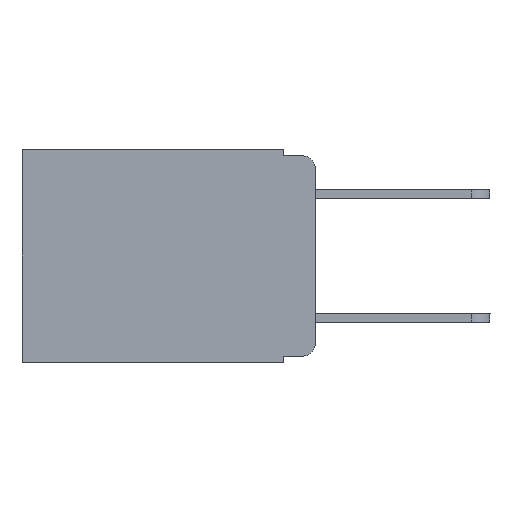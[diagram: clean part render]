
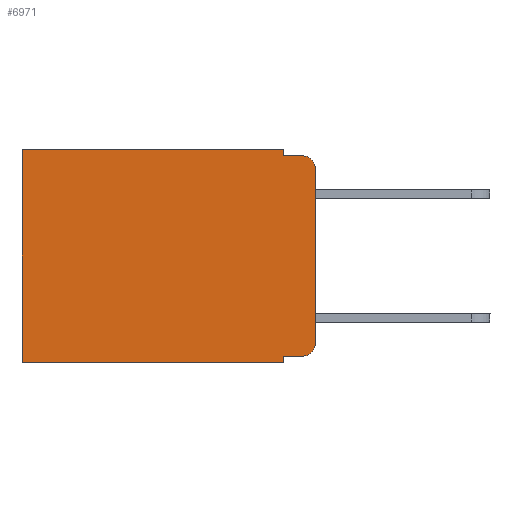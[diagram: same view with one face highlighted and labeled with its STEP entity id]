
A CAD part, left-side view. The second image highlights one B-rep face of the part: STEP entity #6971.
In plain terms, the highlighted planar face has unit normal (-1, 0, 0).
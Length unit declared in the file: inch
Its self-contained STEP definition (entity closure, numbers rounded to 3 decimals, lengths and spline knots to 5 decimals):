
#19 = EDGE_LOOP ( 'NONE', ( #11309, #1333, #9382, #1086, #11175, #11782, #8486, #11681, #6198, #8059 ) ) ;
#22 = CARTESIAN_POINT ( 'NONE',  ( 0.298, 0., -0.343 ) ) ;
#275 = CARTESIAN_POINT ( 'NONE',  ( 0.298, 0., -0.03 ) ) ;
#276 = CARTESIAN_POINT ( 'NONE',  ( 0.298, 0.051, -0.01 ) ) ;
#746 = VERTEX_POINT ( 'NONE', #3378 ) ;
#762 = VECTOR ( 'NONE', #1900, 39.37008 ) ;
#803 = DIRECTION ( 'NONE',  ( -1., 0., 0. ) ) ;
#831 = EDGE_CURVE ( 'NONE', #10962, #7118, #8297, .T. ) ;
#869 = CARTESIAN_POINT ( 'NONE',  ( 0.298, 0.02, -0.313 ) ) ;
#1002 = AXIS2_PLACEMENT_3D ( 'NONE', #869, #2581, #2656 ) ;
#1045 = CARTESIAN_POINT ( 'NONE',  ( 0.298, 0.02, -0.333 ) ) ;
#1086 = ORIENTED_EDGE ( 'NONE', *, *, #831, .F. ) ;
#1136 = PLANE ( 'NONE',  #4852 ) ;
#1247 = DIRECTION ( 'NONE',  ( 0., 0., -1. ) ) ;
#1286 = CARTESIAN_POINT ( 'NONE',  ( 0.298, 0.051, 0. ) ) ;
#1333 = ORIENTED_EDGE ( 'NONE', *, *, #5876, .T. ) ;
#1400 = VECTOR ( 'NONE', #3873, 39.37008 ) ;
#1679 = EDGE_CURVE ( 'NONE', #10876, #7322, #10410, .T. ) ;
#1855 = EDGE_CURVE ( 'NONE', #4520, #7322, #10554, .T. ) ;
#1900 = DIRECTION ( 'NONE',  ( 0., -1., 0. ) ) ;
#2052 = CARTESIAN_POINT ( 'NONE',  ( 0.298, 0.051, -0.343 ) ) ;
#2349 = VERTEX_POINT ( 'NONE', #4841 ) ;
#2581 = DIRECTION ( 'NONE',  ( -1., 0., 0. ) ) ;
#2656 = DIRECTION ( 'NONE',  ( 0., 0., -1. ) ) ;
#2741 = VERTEX_POINT ( 'NONE', #5350 ) ;
#2748 = DIRECTION ( 'NONE',  ( 0., 0., -1. ) ) ;
#2796 = EDGE_CURVE ( 'NONE', #2349, #10876, #5764, .T. ) ;
#2834 = EDGE_CURVE ( 'NONE', #6179, #2741, #4621, .T. ) ;
#2961 = FACE_OUTER_BOUND ( 'NONE', #19, .T. ) ;
#3032 = DIRECTION ( 'NONE',  ( 0., -1., 0. ) ) ;
#3051 = CARTESIAN_POINT ( 'NONE',  ( 0.298, 0., 0. ) ) ;
#3378 = CARTESIAN_POINT ( 'NONE',  ( 0.298, 0.02, -0.01 ) ) ;
#3443 = VECTOR ( 'NONE', #5632, 39.37008 ) ;
#3483 = VECTOR ( 'NONE', #1247, 39.37008 ) ;
#3873 = DIRECTION ( 'NONE',  ( 0., 1., 0. ) ) ;
#4289 = VERTEX_POINT ( 'NONE', #10028 ) ;
#4406 = EDGE_CURVE ( 'NONE', #4289, #2741, #6688, .T. ) ;
#4520 = VERTEX_POINT ( 'NONE', #275 ) ;
#4621 = LINE ( 'NONE', #22, #9868 ) ;
#4659 = CARTESIAN_POINT ( 'NONE',  ( 0.298, 0.051, 0. ) ) ;
#4678 = VECTOR ( 'NONE', #3032, 39.37008 ) ;
#4841 = CARTESIAN_POINT ( 'NONE',  ( 0.298, 0.051, -0.333 ) ) ;
#4852 = AXIS2_PLACEMENT_3D ( 'NONE', #8411, #9332, #10132 ) ;
#4982 = CIRCLE ( 'NONE', #6581, 0.02 ) ;
#5005 = VECTOR ( 'NONE', #9446, 39.37008 ) ;
#5350 = CARTESIAN_POINT ( 'NONE',  ( 0.298, 0.473, -0.343 ) ) ;
#5472 = CARTESIAN_POINT ( 'NONE',  ( 0.298, 0., -0.313 ) ) ;
#5632 = DIRECTION ( 'NONE',  ( 0., 0., -1. ) ) ;
#5764 = LINE ( 'NONE', #8216, #762 ) ;
#5790 = CARTESIAN_POINT ( 'NONE',  ( 0.298, 0.051, 0. ) ) ;
#5876 = EDGE_CURVE ( 'NONE', #4520, #746, #4982, .T. ) ;
#6179 = VERTEX_POINT ( 'NONE', #2052 ) ;
#6198 = ORIENTED_EDGE ( 'NONE', *, *, #2796, .T. ) ;
#6223 = CARTESIAN_POINT ( 'NONE',  ( 0.298, 0.02, -0.03 ) ) ;
#6354 = LINE ( 'NONE', #9318, #1400 ) ;
#6581 = AXIS2_PLACEMENT_3D ( 'NONE', #6223, #803, #9908 ) ;
#6688 = LINE ( 'NONE', #10902, #3443 ) ;
#6971 = ADVANCED_FACE ( 'NONE', ( #2961 ), #1136, .F. ) ;
#7118 = VERTEX_POINT ( 'NONE', #11278 ) ;
#7322 = VERTEX_POINT ( 'NONE', #5472 ) ;
#8059 = ORIENTED_EDGE ( 'NONE', *, *, #1679, .T. ) ;
#8216 = CARTESIAN_POINT ( 'NONE',  ( 0.298, 0.051, -0.333 ) ) ;
#8297 = LINE ( 'NONE', #5790, #3483 ) ;
#8411 = CARTESIAN_POINT ( 'NONE',  ( 0.298, 0., 0. ) ) ;
#8486 = ORIENTED_EDGE ( 'NONE', *, *, #2834, .F. ) ;
#8487 = EDGE_CURVE ( 'NONE', #2349, #6179, #8607, .T. ) ;
#8607 = LINE ( 'NONE', #4659, #9886 ) ;
#9088 = LINE ( 'NONE', #276, #4678 ) ;
#9133 = DIRECTION ( 'NONE',  ( 0., 1., 0. ) ) ;
#9318 = CARTESIAN_POINT ( 'NONE',  ( 0.298, 0., 0. ) ) ;
#9332 = DIRECTION ( 'NONE',  ( 1., 0., 0. ) ) ;
#9382 = ORIENTED_EDGE ( 'NONE', *, *, #10163, .F. ) ;
#9446 = DIRECTION ( 'NONE',  ( 0., 0., -1. ) ) ;
#9868 = VECTOR ( 'NONE', #9133, 39.37008 ) ;
#9886 = VECTOR ( 'NONE', #2748, 39.37008 ) ;
#9908 = DIRECTION ( 'NONE',  ( 0., 0., -1. ) ) ;
#10028 = CARTESIAN_POINT ( 'NONE',  ( 0.298, 0.473, 0. ) ) ;
#10132 = DIRECTION ( 'NONE',  ( 0., 0., -1. ) ) ;
#10163 = EDGE_CURVE ( 'NONE', #7118, #746, #9088, .T. ) ;
#10410 = CIRCLE ( 'NONE', #1002, 0.02 ) ;
#10554 = LINE ( 'NONE', #3051, #5005 ) ;
#10876 = VERTEX_POINT ( 'NONE', #1045 ) ;
#10881 = EDGE_CURVE ( 'NONE', #10962, #4289, #6354, .T. ) ;
#10902 = CARTESIAN_POINT ( 'NONE',  ( 0.298, 0.473, 0. ) ) ;
#10962 = VERTEX_POINT ( 'NONE', #1286 ) ;
#11175 = ORIENTED_EDGE ( 'NONE', *, *, #10881, .T. ) ;
#11278 = CARTESIAN_POINT ( 'NONE',  ( 0.298, 0.051, -0.01 ) ) ;
#11309 = ORIENTED_EDGE ( 'NONE', *, *, #1855, .F. ) ;
#11681 = ORIENTED_EDGE ( 'NONE', *, *, #8487, .F. ) ;
#11782 = ORIENTED_EDGE ( 'NONE', *, *, #4406, .T. ) ;
